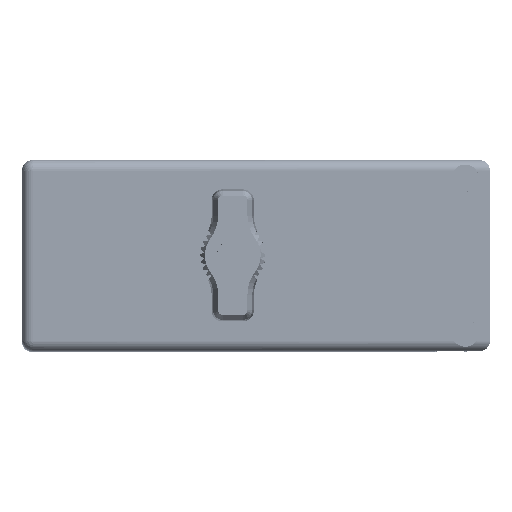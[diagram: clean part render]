
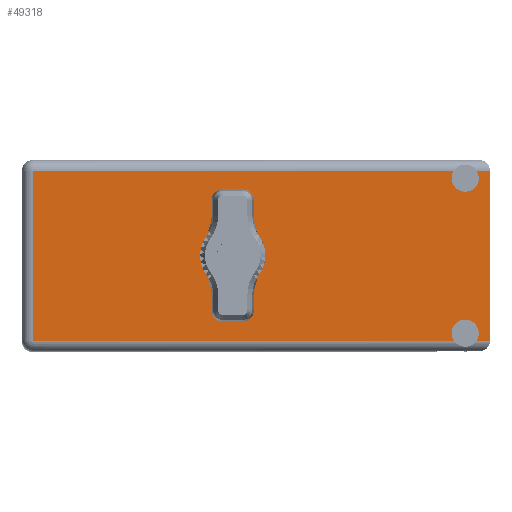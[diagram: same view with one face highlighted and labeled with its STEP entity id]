
A CAD part, top view. The second image highlights one B-rep face of the part: STEP entity #49318.
In plain terms, the highlighted face is planar.
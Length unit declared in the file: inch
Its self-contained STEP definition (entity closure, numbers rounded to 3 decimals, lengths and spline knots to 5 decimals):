
#206 = EDGE_CURVE ( 'NONE', #2635, #16151, #81705, .T. ) ;
#402 = DIRECTION ( 'NONE',  ( 0., 1., 0. ) ) ;
#1518 = PLANE ( 'NONE',  #13082 ) ;
#2485 = CARTESIAN_POINT ( 'NONE',  ( -1.359, 1.675, -0.547 ) ) ;
#2519 = VERTEX_POINT ( 'NONE', #50987 ) ;
#2635 = VERTEX_POINT ( 'NONE', #30192 ) ;
#2664 = DIRECTION ( 'NONE',  ( 0., 0., 1. ) ) ;
#5059 = CARTESIAN_POINT ( 'NONE',  ( 1.659, 1.675, 0.547 ) ) ;
#6131 = CIRCLE ( 'NONE', #21497, 0.0875 ) ;
#7478 = EDGE_CURVE ( 'NONE', #35199, #55743, #12763, .T. ) ;
#7685 = DIRECTION ( 'NONE',  ( 0., 1., 0. ) ) ;
#8613 = CARTESIAN_POINT ( 'NONE',  ( 1.42519, 1.675, 0.547 ) ) ;
#10646 = CARTESIAN_POINT ( 'NONE',  ( -1.289, 1.675, -0.617 ) ) ;
#10972 = CARTESIAN_POINT ( 'NONE',  ( -1.359, 1.675, -0.547 ) ) ;
#12763 = LINE ( 'NONE', #50655, #86102 ) ;
#13082 = AXIS2_PLACEMENT_3D ( 'NONE', #74443, #7685, #21118 ) ;
#15474 = AXIS2_PLACEMENT_3D ( 'NONE', #73917, #402, #47279 ) ;
#16018 = DIRECTION ( 'NONE',  ( 0., 1., 0. ) ) ;
#16151 = VERTEX_POINT ( 'NONE', #20290 ) ;
#17965 = CARTESIAN_POINT ( 'NONE',  ( 1.57281, 1.675, -0.547 ) ) ;
#20290 = CARTESIAN_POINT ( 'NONE',  ( -1.289, 1.675, 0.547 ) ) ;
#20726 = CARTESIAN_POINT ( 'NONE',  ( 0., 1.675, -0.125 ) ) ;
#21118 = DIRECTION ( 'NONE',  ( -1., 0., 0. ) ) ;
#21238 = VERTEX_POINT ( 'NONE', #17965 ) ;
#21497 = AXIS2_PLACEMENT_3D ( 'NONE', #86269, #45045, #38611 ) ;
#21637 = FACE_BOUND ( 'NONE', #28251, .T. ) ;
#22277 = EDGE_CURVE ( 'NONE', #37445, #21238, #6131, .T. ) ;
#23248 = VERTEX_POINT ( 'NONE', #20726 ) ;
#23914 = AXIS2_PLACEMENT_3D ( 'NONE', #67199, #32915, #27076 ) ;
#25118 = LINE ( 'NONE', #2485, #67938 ) ;
#25398 = ORIENTED_EDGE ( 'NONE', *, *, #7478, .F. ) ;
#26434 = ORIENTED_EDGE ( 'NONE', *, *, #83180, .F. ) ;
#26557 = CIRCLE ( 'NONE', #63226, 0.125 ) ;
#27076 = DIRECTION ( 'NONE',  ( 0., 0., 1. ) ) ;
#27086 = CARTESIAN_POINT ( 'NONE',  ( 1.499, 1.675, -0.4125 ) ) ;
#28251 = EDGE_LOOP ( 'NONE', ( #47778, #83811 ) ) ;
#29126 = ORIENTED_EDGE ( 'NONE', *, *, #41669, .F. ) ;
#30192 = CARTESIAN_POINT ( 'NONE',  ( -1.289, 1.675, -0.547 ) ) ;
#30822 = DIRECTION ( 'NONE',  ( 0., 0., 1. ) ) ;
#31976 = DIRECTION ( 'NONE',  ( 1., 0., 0. ) ) ;
#32915 = DIRECTION ( 'NONE',  ( 0., 1., 0. ) ) ;
#35150 = EDGE_CURVE ( 'NONE', #23248, #2519, #26557, .T. ) ;
#35199 = VERTEX_POINT ( 'NONE', #71932 ) ;
#36401 = FACE_OUTER_BOUND ( 'NONE', #52788, .T. ) ;
#37445 = VERTEX_POINT ( 'NONE', #27086 ) ;
#38063 = ORIENTED_EDGE ( 'NONE', *, *, #75910, .T. ) ;
#38611 = DIRECTION ( 'NONE',  ( 0., 0., 1. ) ) ;
#41669 = EDGE_CURVE ( 'NONE', #53361, #37445, #57147, .T. ) ;
#42434 = CARTESIAN_POINT ( 'NONE',  ( 0., 1.675, 0. ) ) ;
#43714 = DIRECTION ( 'NONE',  ( 0., 1., 0. ) ) ;
#44108 = DIRECTION ( 'NONE',  ( 0., 1., 0. ) ) ;
#45045 = DIRECTION ( 'NONE',  ( 0., 1., 0. ) ) ;
#46036 = ORIENTED_EDGE ( 'NONE', *, *, #71007, .F. ) ;
#47279 = DIRECTION ( 'NONE',  ( 0., 0., 1. ) ) ;
#47778 = ORIENTED_EDGE ( 'NONE', *, *, #54860, .F. ) ;
#47950 = CIRCLE ( 'NONE', #48703, 0.0875 ) ;
#48134 = VECTOR ( 'NONE', #31976, 39.37008 ) ;
#48623 = CARTESIAN_POINT ( 'NONE',  ( 0., 1.675, 0. ) ) ;
#48703 = AXIS2_PLACEMENT_3D ( 'NONE', #64280, #44108, #77141 ) ;
#49318 = ADVANCED_FACE ( 'NONE', ( #21637, #36401 ), #1518, .T. ) ;
#49957 = VECTOR ( 'NONE', #63388, 39.37008 ) ;
#49973 = DIRECTION ( 'NONE',  ( 0., 0., 1. ) ) ;
#50113 = VERTEX_POINT ( 'NONE', #64533 ) ;
#50655 = CARTESIAN_POINT ( 'NONE',  ( 1.659, 1.675, 0.617 ) ) ;
#50987 = CARTESIAN_POINT ( 'NONE',  ( 0., 1.675, 0.125 ) ) ;
#52788 = EDGE_LOOP ( 'NONE', ( #79893, #46036, #26434, #57167, #25398, #38063, #75609, #29126, #68429, #76469 ) ) ;
#53361 = VERTEX_POINT ( 'NONE', #69523 ) ;
#54860 = EDGE_CURVE ( 'NONE', #2519, #23248, #85081, .T. ) ;
#55174 = LINE ( 'NONE', #10972, #49957 ) ;
#55743 = VERTEX_POINT ( 'NONE', #62971 ) ;
#57147 = CIRCLE ( 'NONE', #23914, 0.0875 ) ;
#57167 = ORIENTED_EDGE ( 'NONE', *, *, #65905, .T. ) ;
#58072 = VECTOR ( 'NONE', #86093, 39.37008 ) ;
#59896 = VERTEX_POINT ( 'NONE', #72393 ) ;
#61039 = CIRCLE ( 'NONE', #15474, 0.0875 ) ;
#62971 = CARTESIAN_POINT ( 'NONE',  ( 1.659, 1.675, 0.547 ) ) ;
#63226 = AXIS2_PLACEMENT_3D ( 'NONE', #42434, #16018, #49973 ) ;
#63388 = DIRECTION ( 'NONE',  ( -1., 0., 0. ) ) ;
#64280 = CARTESIAN_POINT ( 'NONE',  ( 1.499, 1.675, 0.5 ) ) ;
#64533 = CARTESIAN_POINT ( 'NONE',  ( 1.57281, 1.675, 0.547 ) ) ;
#65905 = EDGE_CURVE ( 'NONE', #50113, #55743, #76437, .T. ) ;
#66192 = CARTESIAN_POINT ( 'NONE',  ( 1.659, 1.675, 0.547 ) ) ;
#67199 = CARTESIAN_POINT ( 'NONE',  ( 1.499, 1.675, -0.5 ) ) ;
#67938 = VECTOR ( 'NONE', #69249, 39.37008 ) ;
#68429 = ORIENTED_EDGE ( 'NONE', *, *, #77836, .T. ) ;
#69249 = DIRECTION ( 'NONE',  ( -1., 0., 0. ) ) ;
#69523 = CARTESIAN_POINT ( 'NONE',  ( 1.42519, 1.675, -0.547 ) ) ;
#70024 = DIRECTION ( 'NONE',  ( 0., 0., 1. ) ) ;
#71007 = EDGE_CURVE ( 'NONE', #59896, #80323, #61039, .T. ) ;
#71932 = CARTESIAN_POINT ( 'NONE',  ( 1.659, 1.675, -0.547 ) ) ;
#72393 = CARTESIAN_POINT ( 'NONE',  ( 1.499, 1.675, 0.4125 ) ) ;
#73917 = CARTESIAN_POINT ( 'NONE',  ( 1.499, 1.675, 0.5 ) ) ;
#74443 = CARTESIAN_POINT ( 'NONE',  ( -1.359, 1.675, -0.617 ) ) ;
#75609 = ORIENTED_EDGE ( 'NONE', *, *, #22277, .F. ) ;
#75910 = EDGE_CURVE ( 'NONE', #35199, #21238, #25118, .T. ) ;
#76437 = LINE ( 'NONE', #5059, #48134 ) ;
#76469 = ORIENTED_EDGE ( 'NONE', *, *, #206, .T. ) ;
#76886 = LINE ( 'NONE', #66192, #58072 ) ;
#77141 = DIRECTION ( 'NONE',  ( 0., 0., 1. ) ) ;
#77836 = EDGE_CURVE ( 'NONE', #53361, #2635, #55174, .T. ) ;
#79893 = ORIENTED_EDGE ( 'NONE', *, *, #85396, .T. ) ;
#80323 = VERTEX_POINT ( 'NONE', #8613 ) ;
#81705 = LINE ( 'NONE', #10646, #85945 ) ;
#83180 = EDGE_CURVE ( 'NONE', #50113, #59896, #47950, .T. ) ;
#83811 = ORIENTED_EDGE ( 'NONE', *, *, #35150, .F. ) ;
#84658 = AXIS2_PLACEMENT_3D ( 'NONE', #48623, #43714, #2664 ) ;
#85081 = CIRCLE ( 'NONE', #84658, 0.125 ) ;
#85396 = EDGE_CURVE ( 'NONE', #16151, #80323, #76886, .T. ) ;
#85945 = VECTOR ( 'NONE', #30822, 39.37008 ) ;
#86093 = DIRECTION ( 'NONE',  ( 1., 0., 0. ) ) ;
#86102 = VECTOR ( 'NONE', #70024, 39.37008 ) ;
#86269 = CARTESIAN_POINT ( 'NONE',  ( 1.499, 1.675, -0.5 ) ) ;
